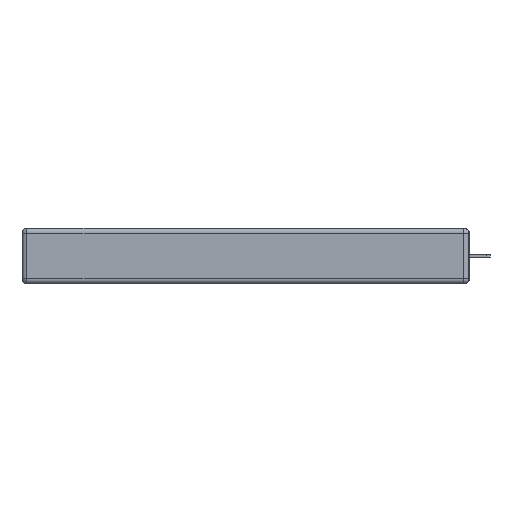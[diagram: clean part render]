
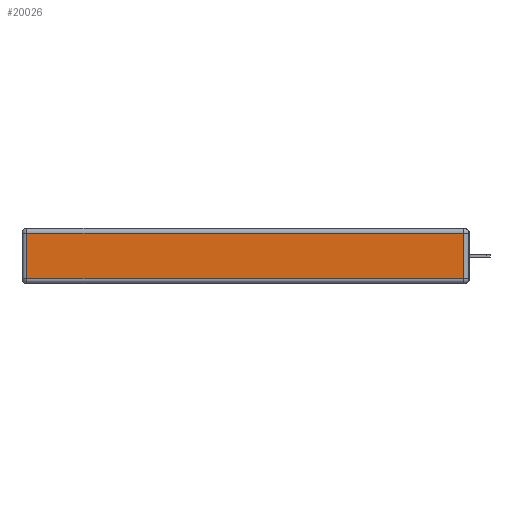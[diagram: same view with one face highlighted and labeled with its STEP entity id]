
A CAD part, left-side view. The second image highlights one B-rep face of the part: STEP entity #20026.
In plain terms, the highlighted planar face has unit normal (-1, 0, 0).
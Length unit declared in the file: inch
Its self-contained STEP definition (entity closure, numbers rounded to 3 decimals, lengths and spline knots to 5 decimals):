
#75 = LINE ( 'NONE', #14173, #20624 ) ;
#2143 = VECTOR ( 'NONE', #5221, 39.37008 ) ;
#2362 = CARTESIAN_POINT ( 'NONE',  ( 0., 0., -0.343 ) ) ;
#2621 = DIRECTION ( 'NONE',  ( 0., 0., -1. ) ) ;
#2830 = ORIENTED_EDGE ( 'NONE', *, *, #16354, .T. ) ;
#4022 = DIRECTION ( 'NONE',  ( 0., 0., 1. ) ) ;
#4588 = EDGE_CURVE ( 'NONE', #17286, #20007, #19440, .T. ) ;
#4690 = CARTESIAN_POINT ( 'NONE',  ( 0., 0.03, -0.03 ) ) ;
#5221 = DIRECTION ( 'NONE',  ( 0., 0., 1. ) ) ;
#6071 = EDGE_CURVE ( 'NONE', #7569, #16766, #75, .T. ) ;
#6898 = CARTESIAN_POINT ( 'NONE',  ( 0., 0.03, -0.343 ) ) ;
#7569 = VERTEX_POINT ( 'NONE', #19761 ) ;
#9783 = EDGE_CURVE ( 'NONE', #20007, #7569, #10772, .T. ) ;
#10268 = ORIENTED_EDGE ( 'NONE', *, *, #9783, .T. ) ;
#10277 = VECTOR ( 'NONE', #2621, 39.37008 ) ;
#10435 = CARTESIAN_POINT ( 'NONE',  ( 0., 2.75, -0.03 ) ) ;
#10772 = LINE ( 'NONE', #15615, #10277 ) ;
#10831 = LINE ( 'NONE', #6898, #2143 ) ;
#12108 = PLANE ( 'NONE',  #15102 ) ;
#12112 = DIRECTION ( 'NONE',  ( 0., 1., 0. ) ) ;
#13667 = CARTESIAN_POINT ( 'NONE',  ( 0., 2.72, -0.03 ) ) ;
#13731 = DIRECTION ( 'NONE',  ( -1., 0., 0. ) ) ;
#14173 = CARTESIAN_POINT ( 'NONE',  ( 0., 0., -0.313 ) ) ;
#14495 = EDGE_LOOP ( 'NONE', ( #17684, #2830, #15253, #10268 ) ) ;
#14636 = FACE_OUTER_BOUND ( 'NONE', #14495, .T. ) ;
#15102 = AXIS2_PLACEMENT_3D ( 'NONE', #2362, #13731, #4022 ) ;
#15253 = ORIENTED_EDGE ( 'NONE', *, *, #4588, .T. ) ;
#15615 = CARTESIAN_POINT ( 'NONE',  ( 0., 2.72, -0.343 ) ) ;
#15794 = DIRECTION ( 'NONE',  ( 0., -1., 0. ) ) ;
#16354 = EDGE_CURVE ( 'NONE', #16766, #17286, #10831, .T. ) ;
#16766 = VERTEX_POINT ( 'NONE', #19436 ) ;
#17286 = VERTEX_POINT ( 'NONE', #4690 ) ;
#17684 = ORIENTED_EDGE ( 'NONE', *, *, #6071, .T. ) ;
#18944 = VECTOR ( 'NONE', #12112, 39.37008 ) ;
#19436 = CARTESIAN_POINT ( 'NONE',  ( 0., 0.03, -0.313 ) ) ;
#19440 = LINE ( 'NONE', #10435, #18944 ) ;
#19761 = CARTESIAN_POINT ( 'NONE',  ( 0., 2.72, -0.313 ) ) ;
#20007 = VERTEX_POINT ( 'NONE', #13667 ) ;
#20026 = ADVANCED_FACE ( 'NONE', ( #14636 ), #12108, .T. ) ;
#20624 = VECTOR ( 'NONE', #15794, 39.37008 ) ;
